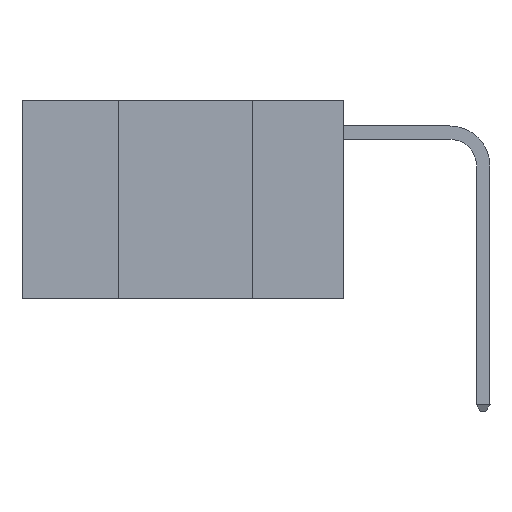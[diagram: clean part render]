
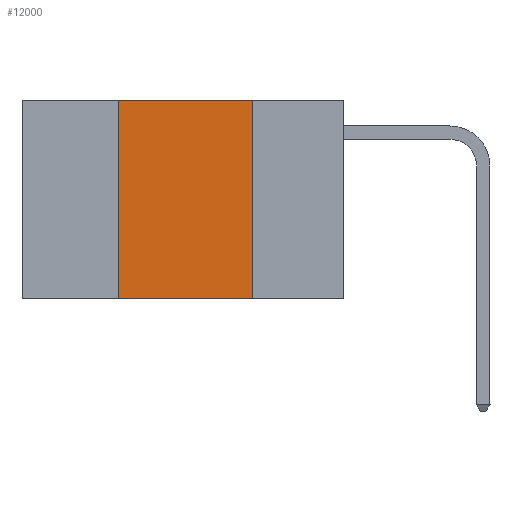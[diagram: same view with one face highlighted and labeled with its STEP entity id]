
A CAD part, left-side view. The second image highlights one B-rep face of the part: STEP entity #12000.
In plain terms, the highlighted planar face has unit normal (-1, 0, 0).
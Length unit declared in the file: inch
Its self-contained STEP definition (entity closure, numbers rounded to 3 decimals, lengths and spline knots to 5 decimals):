
#818 = EDGE_CURVE ( 'NONE', #12822, #27602, #3985, .T. ) ;
#1794 = CARTESIAN_POINT ( 'NONE',  ( 0., 0.17, -0.37 ) ) ;
#2088 = CARTESIAN_POINT ( 'NONE',  ( 0., 0.17, 0. ) ) ;
#2246 = CARTESIAN_POINT ( 'NONE',  ( 0., 0.42, 0. ) ) ;
#2831 = EDGE_CURVE ( 'NONE', #26312, #12822, #5106, .T. ) ;
#3985 = LINE ( 'NONE', #17370, #16527 ) ;
#4420 = LINE ( 'NONE', #2246, #9474 ) ;
#5106 = LINE ( 'NONE', #25445, #27715 ) ;
#6426 = EDGE_CURVE ( 'NONE', #19811, #27602, #17129, .T. ) ;
#7192 = ORIENTED_EDGE ( 'NONE', *, *, #9611, .F. ) ;
#8565 = CARTESIAN_POINT ( 'NONE',  ( 0., 0.6, 0. ) ) ;
#9117 = AXIS2_PLACEMENT_3D ( 'NONE', #8565, #16881, #25732 ) ;
#9474 = VECTOR ( 'NONE', #19988, 39.37008 ) ;
#9611 = EDGE_CURVE ( 'NONE', #19811, #26312, #4420, .T. ) ;
#10068 = ORIENTED_EDGE ( 'NONE', *, *, #2831, .F. ) ;
#10574 = DIRECTION ( 'NONE',  ( 0., -1., 0. ) ) ;
#11481 = CARTESIAN_POINT ( 'NONE',  ( 0., 0.42, 0. ) ) ;
#12000 = ADVANCED_FACE ( 'NONE', ( #15121 ), #19471, .F. ) ;
#12069 = ORIENTED_EDGE ( 'NONE', *, *, #818, .F. ) ;
#12481 = EDGE_LOOP ( 'NONE', ( #12069, #10068, #7192, #26106 ) ) ;
#12822 = VERTEX_POINT ( 'NONE', #2088 ) ;
#12863 = DIRECTION ( 'NONE',  ( 0., 0., -1. ) ) ;
#14406 = DIRECTION ( 'NONE',  ( 0., -1., 0. ) ) ;
#15121 = FACE_OUTER_BOUND ( 'NONE', #12481, .T. ) ;
#16527 = VECTOR ( 'NONE', #12863, 39.37008 ) ;
#16881 = DIRECTION ( 'NONE',  ( 1., 0., 0. ) ) ;
#16930 = CARTESIAN_POINT ( 'NONE',  ( 0., 0.42, -0.37 ) ) ;
#17129 = LINE ( 'NONE', #19713, #21726 ) ;
#17370 = CARTESIAN_POINT ( 'NONE',  ( 0., 0.17, 0. ) ) ;
#19471 = PLANE ( 'NONE',  #9117 ) ;
#19713 = CARTESIAN_POINT ( 'NONE',  ( 0., 0.6, -0.37 ) ) ;
#19811 = VERTEX_POINT ( 'NONE', #16930 ) ;
#19988 = DIRECTION ( 'NONE',  ( 0., 0., 1. ) ) ;
#21726 = VECTOR ( 'NONE', #10574, 39.37008 ) ;
#25445 = CARTESIAN_POINT ( 'NONE',  ( 0., 0.6, 0. ) ) ;
#25732 = DIRECTION ( 'NONE',  ( 0., 0., -1. ) ) ;
#26106 = ORIENTED_EDGE ( 'NONE', *, *, #6426, .T. ) ;
#26312 = VERTEX_POINT ( 'NONE', #11481 ) ;
#27602 = VERTEX_POINT ( 'NONE', #1794 ) ;
#27715 = VECTOR ( 'NONE', #14406, 39.37008 ) ;
